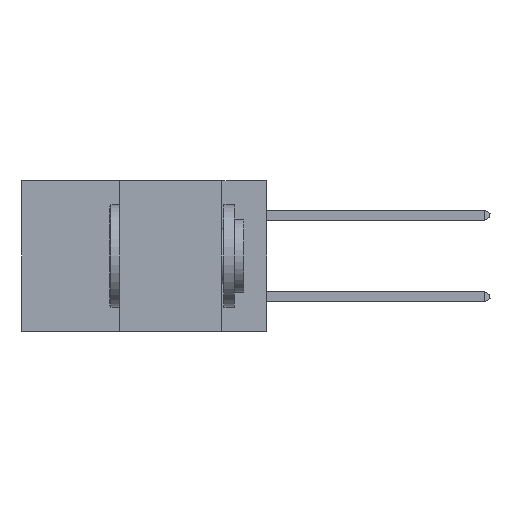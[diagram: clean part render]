
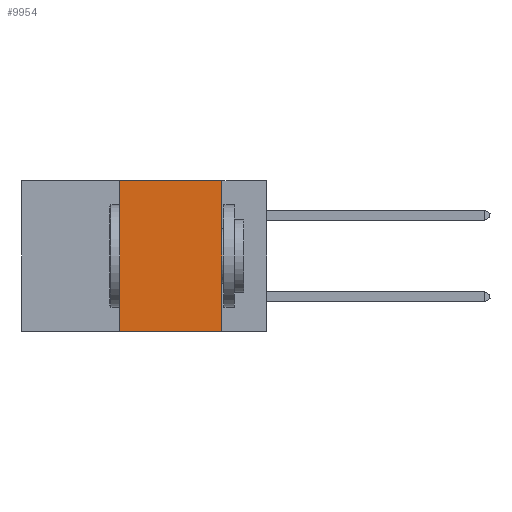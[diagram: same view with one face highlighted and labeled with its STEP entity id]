
A CAD part, left-side view. The second image highlights one B-rep face of the part: STEP entity #9954.
In plain terms, the highlighted planar face has unit normal (-1, 0, 0).
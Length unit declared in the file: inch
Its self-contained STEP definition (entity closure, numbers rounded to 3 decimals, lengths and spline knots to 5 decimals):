
#137 = CARTESIAN_POINT ( 'NONE',  ( 0., 0.6, 0. ) ) ;
#1174 = CARTESIAN_POINT ( 'NONE',  ( 0., 0.11, -0.37 ) ) ;
#1814 = ORIENTED_EDGE ( 'NONE', *, *, #16736, .F. ) ;
#1873 = ORIENTED_EDGE ( 'NONE', *, *, #8703, .T. ) ;
#2249 = CARTESIAN_POINT ( 'NONE',  ( 0., 0.6, 0. ) ) ;
#2866 = EDGE_LOOP ( 'NONE', ( #6523, #1814, #12563, #1873 ) ) ;
#3006 = PLANE ( 'NONE',  #16720 ) ;
#3303 = VERTEX_POINT ( 'NONE', #1174 ) ;
#3464 = VERTEX_POINT ( 'NONE', #11720 ) ;
#3745 = DIRECTION ( 'NONE',  ( 0., 0., 1. ) ) ;
#4006 = CARTESIAN_POINT ( 'NONE',  ( 0., 0.11, 0. ) ) ;
#4419 = VECTOR ( 'NONE', #3745, 39.37008 ) ;
#4479 = DIRECTION ( 'NONE',  ( 1., 0., 0. ) ) ;
#4829 = DIRECTION ( 'NONE',  ( 0., 0., -1. ) ) ;
#6523 = ORIENTED_EDGE ( 'NONE', *, *, #6965, .F. ) ;
#6548 = DIRECTION ( 'NONE',  ( 0., -1., 0. ) ) ;
#6647 = LINE ( 'NONE', #10623, #8496 ) ;
#6656 = EDGE_CURVE ( 'NONE', #3464, #11827, #11444, .T. ) ;
#6965 = EDGE_CURVE ( 'NONE', #13176, #3303, #6647, .T. ) ;
#8496 = VECTOR ( 'NONE', #4829, 39.37008 ) ;
#8703 = EDGE_CURVE ( 'NONE', #3464, #3303, #12086, .T. ) ;
#9954 = ADVANCED_FACE ( 'NONE', ( #17003 ), #3006, .F. ) ;
#10313 = DIRECTION ( 'NONE',  ( 0., 0., -1. ) ) ;
#10355 = VECTOR ( 'NONE', #6548, 39.37008 ) ;
#10623 = CARTESIAN_POINT ( 'NONE',  ( 0., 0.11, 0. ) ) ;
#10821 = LINE ( 'NONE', #2249, #10355 ) ;
#11206 = DIRECTION ( 'NONE',  ( 0., -1., 0. ) ) ;
#11444 = LINE ( 'NONE', #12445, #4419 ) ;
#11720 = CARTESIAN_POINT ( 'NONE',  ( 0., 0.36, -0.37 ) ) ;
#11827 = VERTEX_POINT ( 'NONE', #14302 ) ;
#12086 = LINE ( 'NONE', #18552, #13198 ) ;
#12445 = CARTESIAN_POINT ( 'NONE',  ( 0., 0.36, 0. ) ) ;
#12563 = ORIENTED_EDGE ( 'NONE', *, *, #6656, .F. ) ;
#13176 = VERTEX_POINT ( 'NONE', #4006 ) ;
#13198 = VECTOR ( 'NONE', #11206, 39.37008 ) ;
#14302 = CARTESIAN_POINT ( 'NONE',  ( 0., 0.36, 0. ) ) ;
#16720 = AXIS2_PLACEMENT_3D ( 'NONE', #137, #4479, #10313 ) ;
#16736 = EDGE_CURVE ( 'NONE', #11827, #13176, #10821, .T. ) ;
#17003 = FACE_OUTER_BOUND ( 'NONE', #2866, .T. ) ;
#18552 = CARTESIAN_POINT ( 'NONE',  ( 0., 0.6, -0.37 ) ) ;
